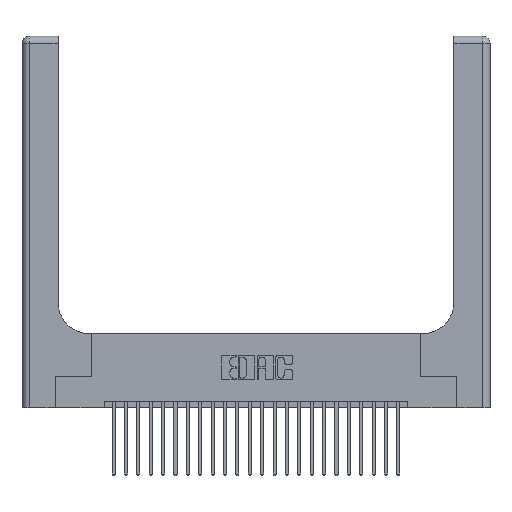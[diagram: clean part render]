
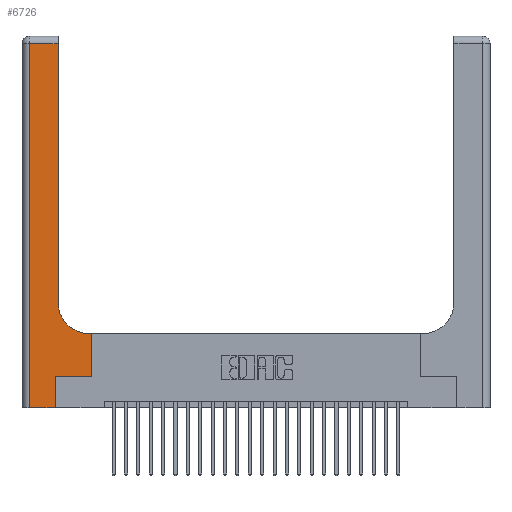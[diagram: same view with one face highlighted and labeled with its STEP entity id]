
A CAD part, top view. The second image highlights one B-rep face of the part: STEP entity #6726.
In plain terms, the highlighted planar face has unit normal (0, 0, 1).
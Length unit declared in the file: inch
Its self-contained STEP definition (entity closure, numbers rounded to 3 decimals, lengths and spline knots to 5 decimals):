
#532 = CIRCLE ( 'NONE', #3925, 0.25 ) ;
#811 = DIRECTION ( 'NONE',  ( 0., 0., -1. ) ) ;
#835 = ORIENTED_EDGE ( 'NONE', *, *, #18051, .T. ) ;
#2460 = VERTEX_POINT ( 'NONE', #4123 ) ;
#3125 = DIRECTION ( 'NONE',  ( 1., 0., 0. ) ) ;
#3257 = CARTESIAN_POINT ( 'NONE',  ( 0.2915, 0.85, 0.37 ) ) ;
#3856 = CARTESIAN_POINT ( 'NONE',  ( 0.5585, 0.6, 0.37 ) ) ;
#3925 = AXIS2_PLACEMENT_3D ( 'NONE', #13383, #811, #15387 ) ;
#4123 = CARTESIAN_POINT ( 'NONE',  ( 0.5585, 0.25, 0.37 ) ) ;
#4308 = CARTESIAN_POINT ( 'NONE',  ( 0., 3., 0.37 ) ) ;
#5010 = VERTEX_POINT ( 'NONE', #6282 ) ;
#5456 = LINE ( 'NONE', #20578, #26329 ) ;
#6163 = VECTOR ( 'NONE', #21195, 39.37008 ) ;
#6282 = CARTESIAN_POINT ( 'NONE',  ( 0.269, 0., 0.37 ) ) ;
#6351 = DIRECTION ( 'NONE',  ( 0., 1., 0. ) ) ;
#6406 = DIRECTION ( 'NONE',  ( 0., 0., -1. ) ) ;
#6581 = VERTEX_POINT ( 'NONE', #3856 ) ;
#6726 = ADVANCED_FACE ( 'NONE', ( #24728 ), #16653, .F. ) ;
#7027 = CARTESIAN_POINT ( 'NONE',  ( 0.2915, 0.6, 0.37 ) ) ;
#7777 = CARTESIAN_POINT ( 'NONE',  ( 0.06, 3., 0.37 ) ) ;
#7950 = CARTESIAN_POINT ( 'NONE',  ( 0.06, 2.94, 0.37 ) ) ;
#8560 = DIRECTION ( 'NONE',  ( 0., 1., 0. ) ) ;
#9005 = CARTESIAN_POINT ( 'NONE',  ( 0., 2.94, 0.37 ) ) ;
#9278 = VERTEX_POINT ( 'NONE', #13906 ) ;
#9382 = LINE ( 'NONE', #9384, #20123 ) ;
#9384 = CARTESIAN_POINT ( 'NONE',  ( 0.269, 0.25, 0.37 ) ) ;
#9392 = LINE ( 'NONE', #7777, #19496 ) ;
#9870 = DIRECTION ( 'NONE',  ( 0., -1., 0. ) ) ;
#10407 = ORIENTED_EDGE ( 'NONE', *, *, #23901, .T. ) ;
#10541 = CARTESIAN_POINT ( 'NONE',  ( 0.269, 0., 0.37 ) ) ;
#10608 = VECTOR ( 'NONE', #17856, 39.37008 ) ;
#11932 = VERTEX_POINT ( 'NONE', #16864 ) ;
#12084 = LINE ( 'NONE', #9005, #18050 ) ;
#12361 = LINE ( 'NONE', #7027, #6163 ) ;
#13375 = VERTEX_POINT ( 'NONE', #3257 ) ;
#13383 = CARTESIAN_POINT ( 'NONE',  ( 0.5415, 0.85, 0.37 ) ) ;
#13477 = ORIENTED_EDGE ( 'NONE', *, *, #15238, .T. ) ;
#13558 = DIRECTION ( 'NONE',  ( 0., 1., 0. ) ) ;
#13906 = CARTESIAN_POINT ( 'NONE',  ( 0.2915, 2.94, 0.37 ) ) ;
#14386 = EDGE_CURVE ( 'NONE', #2460, #6581, #18853, .T. ) ;
#15174 = ORIENTED_EDGE ( 'NONE', *, *, #14386, .T. ) ;
#15238 = EDGE_CURVE ( 'NONE', #11932, #5010, #21899, .T. ) ;
#15325 = VERTEX_POINT ( 'NONE', #26107 ) ;
#15387 = DIRECTION ( 'NONE',  ( 1., 0., 0. ) ) ;
#15593 = EDGE_LOOP ( 'NONE', ( #10407, #20950, #17182, #13477, #835, #21940, #15174, #19953, #21125 ) ) ;
#16653 = PLANE ( 'NONE',  #19989 ) ;
#16864 = CARTESIAN_POINT ( 'NONE',  ( 0.06, 0., 0.37 ) ) ;
#17182 = ORIENTED_EDGE ( 'NONE', *, *, #17257, .T. ) ;
#17257 = EDGE_CURVE ( 'NONE', #19214, #11932, #9392, .T. ) ;
#17856 = DIRECTION ( 'NONE',  ( 1., 0., 0. ) ) ;
#18050 = VECTOR ( 'NONE', #23060, 39.37008 ) ;
#18051 = EDGE_CURVE ( 'NONE', #5010, #15325, #21302, .T. ) ;
#18853 = LINE ( 'NONE', #23458, #24132 ) ;
#19214 = VERTEX_POINT ( 'NONE', #7950 ) ;
#19496 = VECTOR ( 'NONE', #9870, 39.37008 ) ;
#19953 = ORIENTED_EDGE ( 'NONE', *, *, #21421, .T. ) ;
#19989 = AXIS2_PLACEMENT_3D ( 'NONE', #4308, #6406, #20631 ) ;
#20123 = VECTOR ( 'NONE', #3125, 39.37008 ) ;
#20578 = CARTESIAN_POINT ( 'NONE',  ( 0.2915, 3., 0.37 ) ) ;
#20631 = DIRECTION ( 'NONE',  ( -1., 0., 0. ) ) ;
#20686 = VECTOR ( 'NONE', #8560, 39.37008 ) ;
#20705 = EDGE_CURVE ( 'NONE', #9278, #19214, #12084, .T. ) ;
#20920 = VERTEX_POINT ( 'NONE', #23654 ) ;
#20950 = ORIENTED_EDGE ( 'NONE', *, *, #20705, .T. ) ;
#21125 = ORIENTED_EDGE ( 'NONE', *, *, #21425, .T. ) ;
#21195 = DIRECTION ( 'NONE',  ( -1., 0., 0. ) ) ;
#21302 = LINE ( 'NONE', #10541, #20686 ) ;
#21421 = EDGE_CURVE ( 'NONE', #6581, #20920, #12361, .T. ) ;
#21425 = EDGE_CURVE ( 'NONE', #20920, #13375, #532, .T. ) ;
#21899 = LINE ( 'NONE', #25842, #10608 ) ;
#21940 = ORIENTED_EDGE ( 'NONE', *, *, #24179, .T. ) ;
#23060 = DIRECTION ( 'NONE',  ( -1., 0., 0. ) ) ;
#23458 = CARTESIAN_POINT ( 'NONE',  ( 0.5585, 0.25, 0.37 ) ) ;
#23654 = CARTESIAN_POINT ( 'NONE',  ( 0.5415, 0.6, 0.37 ) ) ;
#23901 = EDGE_CURVE ( 'NONE', #13375, #9278, #5456, .T. ) ;
#24132 = VECTOR ( 'NONE', #13558, 39.37008 ) ;
#24179 = EDGE_CURVE ( 'NONE', #15325, #2460, #9382, .T. ) ;
#24728 = FACE_OUTER_BOUND ( 'NONE', #15593, .T. ) ;
#25842 = CARTESIAN_POINT ( 'NONE',  ( 0., 0., 0.37 ) ) ;
#26107 = CARTESIAN_POINT ( 'NONE',  ( 0.269, 0.25, 0.37 ) ) ;
#26329 = VECTOR ( 'NONE', #6351, 39.37008 ) ;
